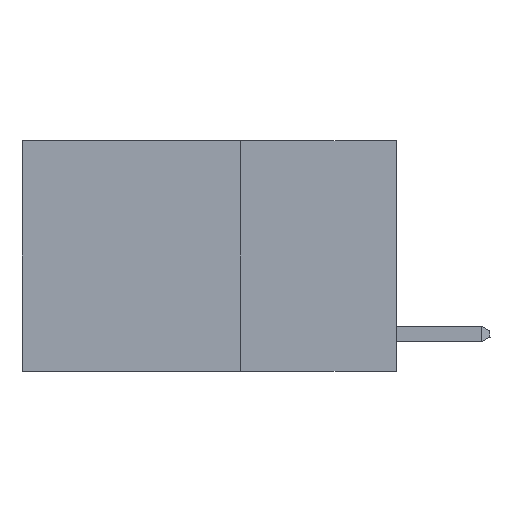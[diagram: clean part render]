
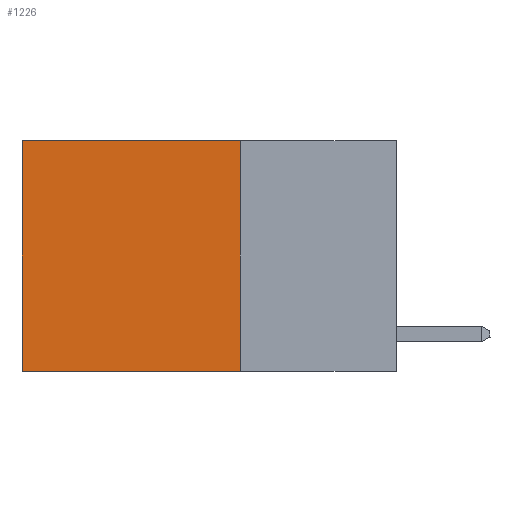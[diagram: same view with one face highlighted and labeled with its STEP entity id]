
A CAD part, left-side view. The second image highlights one B-rep face of the part: STEP entity #1226.
In plain terms, the highlighted planar face has unit normal (-1, 0, 0).
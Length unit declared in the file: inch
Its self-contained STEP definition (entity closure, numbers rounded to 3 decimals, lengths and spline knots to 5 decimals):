
#146 = DIRECTION ( 'NONE',  ( 0., 0., -1. ) ) ;
#565 = CARTESIAN_POINT ( 'NONE',  ( 0.2625, 0.6, -0.37 ) ) ;
#1179 = EDGE_CURVE ( 'NONE', #5132, #7623, #8718, .T. ) ;
#1226 = ADVANCED_FACE ( 'NONE', ( #8292 ), #12308, .F. ) ;
#1231 = VECTOR ( 'NONE', #146, 39.37008 ) ;
#1442 = LINE ( 'NONE', #5976, #9096 ) ;
#1921 = DIRECTION ( 'NONE',  ( 0., 0., -1. ) ) ;
#2690 = EDGE_CURVE ( 'NONE', #15175, #14282, #8034, .T. ) ;
#2810 = CARTESIAN_POINT ( 'NONE',  ( 0.2625, 0.25, 0. ) ) ;
#3406 = EDGE_CURVE ( 'NONE', #7623, #14282, #4863, .T. ) ;
#3792 = EDGE_LOOP ( 'NONE', ( #14918, #8602, #14071, #14764 ) ) ;
#4021 = VECTOR ( 'NONE', #5630, 39.37008 ) ;
#4257 = CARTESIAN_POINT ( 'NONE',  ( 0.2625, 0.25, 0. ) ) ;
#4863 = LINE ( 'NONE', #15031, #1231 ) ;
#5132 = VERTEX_POINT ( 'NONE', #10738 ) ;
#5612 = DIRECTION ( 'NONE',  ( 1., 0., 0. ) ) ;
#5630 = DIRECTION ( 'NONE',  ( 0., 1., 0. ) ) ;
#5976 = CARTESIAN_POINT ( 'NONE',  ( 0.2625, 0.25, 0. ) ) ;
#6235 = CARTESIAN_POINT ( 'NONE',  ( 0.2625, 0.25, -0.37 ) ) ;
#7623 = VERTEX_POINT ( 'NONE', #12295 ) ;
#8034 = LINE ( 'NONE', #13684, #4021 ) ;
#8292 = FACE_OUTER_BOUND ( 'NONE', #3792, .T. ) ;
#8602 = ORIENTED_EDGE ( 'NONE', *, *, #2690, .F. ) ;
#8718 = LINE ( 'NONE', #2810, #12702 ) ;
#9096 = VECTOR ( 'NONE', #1921, 39.37008 ) ;
#9153 = AXIS2_PLACEMENT_3D ( 'NONE', #4257, #5612, #15034 ) ;
#10402 = EDGE_CURVE ( 'NONE', #5132, #15175, #1442, .T. ) ;
#10738 = CARTESIAN_POINT ( 'NONE',  ( 0.2625, 0.25, 0. ) ) ;
#12251 = DIRECTION ( 'NONE',  ( 0., 1., 0. ) ) ;
#12295 = CARTESIAN_POINT ( 'NONE',  ( 0.2625, 0.6, 0. ) ) ;
#12308 = PLANE ( 'NONE',  #9153 ) ;
#12702 = VECTOR ( 'NONE', #12251, 39.37008 ) ;
#13684 = CARTESIAN_POINT ( 'NONE',  ( 0.2625, 0.25, -0.37 ) ) ;
#14071 = ORIENTED_EDGE ( 'NONE', *, *, #10402, .F. ) ;
#14282 = VERTEX_POINT ( 'NONE', #565 ) ;
#14764 = ORIENTED_EDGE ( 'NONE', *, *, #1179, .T. ) ;
#14918 = ORIENTED_EDGE ( 'NONE', *, *, #3406, .T. ) ;
#15031 = CARTESIAN_POINT ( 'NONE',  ( 0.2625, 0.6, 0. ) ) ;
#15034 = DIRECTION ( 'NONE',  ( 0., 0., -1. ) ) ;
#15175 = VERTEX_POINT ( 'NONE', #6235 ) ;
